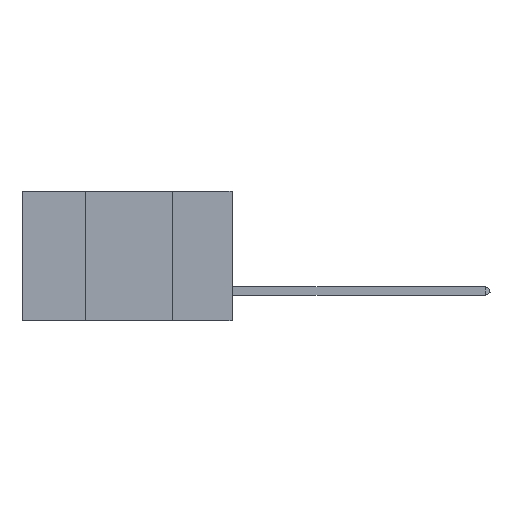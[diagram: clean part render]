
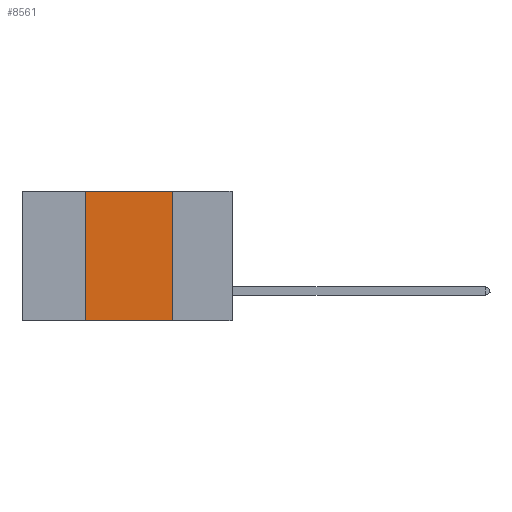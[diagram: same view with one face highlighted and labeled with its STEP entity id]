
A CAD part, left-side view. The second image highlights one B-rep face of the part: STEP entity #8561.
In plain terms, the highlighted planar face has unit normal (-1, 0, 0).
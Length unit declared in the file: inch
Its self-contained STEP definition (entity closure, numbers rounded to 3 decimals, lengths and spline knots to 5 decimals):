
#440 = CARTESIAN_POINT ( 'NONE',  ( 0., 0.42, 0. ) ) ;
#1386 = VERTEX_POINT ( 'NONE', #15234 ) ;
#1483 = EDGE_LOOP ( 'NONE', ( #5978, #17361, #13400, #8640 ) ) ;
#1634 = LINE ( 'NONE', #8031, #20981 ) ;
#2159 = CARTESIAN_POINT ( 'NONE',  ( 0., 0.42, -0.37 ) ) ;
#4402 = CARTESIAN_POINT ( 'NONE',  ( 0., 0.6, 0. ) ) ;
#5549 = EDGE_CURVE ( 'NONE', #7458, #6646, #10028, .T. ) ;
#5978 = ORIENTED_EDGE ( 'NONE', *, *, #22430, .F. ) ;
#6361 = DIRECTION ( 'NONE',  ( 1., 0., 0. ) ) ;
#6646 = VERTEX_POINT ( 'NONE', #16452 ) ;
#7240 = CARTESIAN_POINT ( 'NONE',  ( 0., 0.6, 0. ) ) ;
#7458 = VERTEX_POINT ( 'NONE', #2159 ) ;
#7525 = LINE ( 'NONE', #14653, #12251 ) ;
#8024 = DIRECTION ( 'NONE',  ( 0., 0., 1. ) ) ;
#8031 = CARTESIAN_POINT ( 'NONE',  ( 0., 0.6, -0.37 ) ) ;
#8272 = DIRECTION ( 'NONE',  ( 0., 0., -1. ) ) ;
#8561 = ADVANCED_FACE ( 'NONE', ( #10181 ), #15559, .F. ) ;
#8640 = ORIENTED_EDGE ( 'NONE', *, *, #12234, .T. ) ;
#8889 = VECTOR ( 'NONE', #8024, 39.37008 ) ;
#8911 = CARTESIAN_POINT ( 'NONE',  ( 0., 0.17, 0. ) ) ;
#10028 = LINE ( 'NONE', #440, #8889 ) ;
#10181 = FACE_OUTER_BOUND ( 'NONE', #1483, .T. ) ;
#10185 = VECTOR ( 'NONE', #18202, 39.37008 ) ;
#12234 = EDGE_CURVE ( 'NONE', #7458, #1386, #1634, .T. ) ;
#12251 = VECTOR ( 'NONE', #22261, 39.37008 ) ;
#13400 = ORIENTED_EDGE ( 'NONE', *, *, #5549, .F. ) ;
#14260 = DIRECTION ( 'NONE',  ( 0., -1., 0. ) ) ;
#14653 = CARTESIAN_POINT ( 'NONE',  ( 0., 0.17, 0. ) ) ;
#15234 = CARTESIAN_POINT ( 'NONE',  ( 0., 0.17, -0.37 ) ) ;
#15427 = VERTEX_POINT ( 'NONE', #8911 ) ;
#15559 = PLANE ( 'NONE',  #19469 ) ;
#16452 = CARTESIAN_POINT ( 'NONE',  ( 0., 0.42, 0. ) ) ;
#17361 = ORIENTED_EDGE ( 'NONE', *, *, #21737, .F. ) ;
#18202 = DIRECTION ( 'NONE',  ( 0., -1., 0. ) ) ;
#19469 = AXIS2_PLACEMENT_3D ( 'NONE', #4402, #6361, #8272 ) ;
#20744 = LINE ( 'NONE', #7240, #10185 ) ;
#20981 = VECTOR ( 'NONE', #14260, 39.37008 ) ;
#21737 = EDGE_CURVE ( 'NONE', #6646, #15427, #20744, .T. ) ;
#22261 = DIRECTION ( 'NONE',  ( 0., 0., -1. ) ) ;
#22430 = EDGE_CURVE ( 'NONE', #15427, #1386, #7525, .T. ) ;
